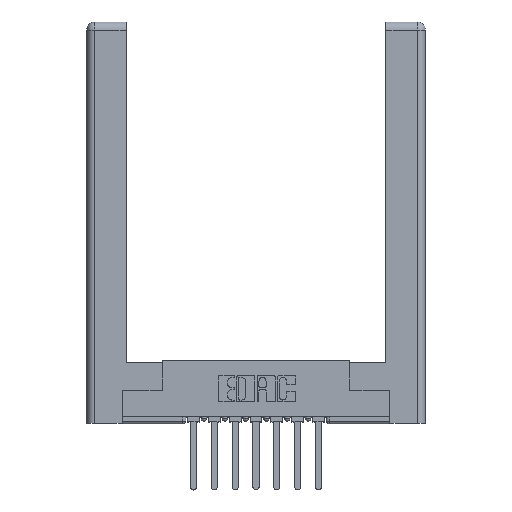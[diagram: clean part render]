
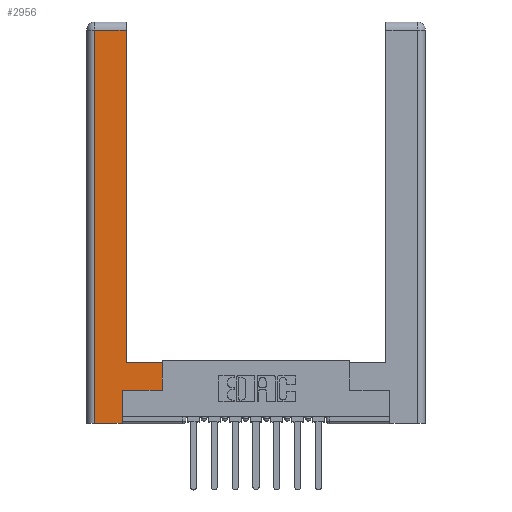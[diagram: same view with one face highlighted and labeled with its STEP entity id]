
A CAD part, top view. The second image highlights one B-rep face of the part: STEP entity #2956.
In plain terms, the highlighted planar face has unit normal (0, 0, 1).
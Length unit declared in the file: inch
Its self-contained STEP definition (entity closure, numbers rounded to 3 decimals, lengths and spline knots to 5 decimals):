
#50 = DIRECTION ( 'NONE',  ( -1., 0., 0. ) ) ;
#137 = DIRECTION ( 'NONE',  ( 0., 1., 0. ) ) ;
#250 = CARTESIAN_POINT ( 'NONE',  ( 0.265, 0.245, 0. ) ) ;
#469 = CARTESIAN_POINT ( 'NONE',  ( 0.295, 2.94, 0. ) ) ;
#1010 = VERTEX_POINT ( 'NONE', #1948 ) ;
#1033 = ORIENTED_EDGE ( 'NONE', *, *, #1061, .T. ) ;
#1061 = EDGE_CURVE ( 'NONE', #2699, #8455, #7199, .T. ) ;
#1087 = VERTEX_POINT ( 'NONE', #6345 ) ;
#1153 = CARTESIAN_POINT ( 'NONE',  ( 0.0615, 0., 0. ) ) ;
#1284 = CARTESIAN_POINT ( 'NONE',  ( 0.265, 0., 0. ) ) ;
#1726 = DIRECTION ( 'NONE',  ( 1., 0., 0. ) ) ;
#1829 = ORIENTED_EDGE ( 'NONE', *, *, #2673, .T. ) ;
#1948 = CARTESIAN_POINT ( 'NONE',  ( 0.295, 0.45, 0. ) ) ;
#2093 = VECTOR ( 'NONE', #1726, 39.37008 ) ;
#2288 = DIRECTION ( 'NONE',  ( -1., 0., 0. ) ) ;
#2411 = LINE ( 'NONE', #10979, #10341 ) ;
#2460 = VECTOR ( 'NONE', #11695, 39.37008 ) ;
#2673 = EDGE_CURVE ( 'NONE', #10472, #10853, #9185, .T. ) ;
#2699 = VERTEX_POINT ( 'NONE', #469 ) ;
#2748 = CARTESIAN_POINT ( 'NONE',  ( 0.265, 0.245, 0. ) ) ;
#2874 = VECTOR ( 'NONE', #50, 39.37008 ) ;
#2956 = ADVANCED_FACE ( 'NONE', ( #8522 ), #5592, .F. ) ;
#3079 = CARTESIAN_POINT ( 'NONE',  ( 0.295, 0.45, 0. ) ) ;
#3180 = EDGE_CURVE ( 'NONE', #10853, #1087, #10027, .T. ) ;
#3404 = DIRECTION ( 'NONE',  ( 0., 1., 0. ) ) ;
#3764 = ORIENTED_EDGE ( 'NONE', *, *, #3180, .T. ) ;
#3773 = CARTESIAN_POINT ( 'NONE',  ( 0.565, 0.245, 0. ) ) ;
#4238 = VECTOR ( 'NONE', #2288, 39.37008 ) ;
#4495 = DIRECTION ( 'NONE',  ( 0., 1., 0. ) ) ;
#4702 = AXIS2_PLACEMENT_3D ( 'NONE', #13193, #13067, #6669 ) ;
#4925 = LINE ( 'NONE', #6634, #10944 ) ;
#5345 = ORIENTED_EDGE ( 'NONE', *, *, #11799, .T. ) ;
#5592 = PLANE ( 'NONE',  #4702 ) ;
#5763 = ORIENTED_EDGE ( 'NONE', *, *, #10010, .T. ) ;
#6034 = LINE ( 'NONE', #1153, #2460 ) ;
#6285 = DIRECTION ( 'NONE',  ( 1., 0., 0. ) ) ;
#6345 = CARTESIAN_POINT ( 'NONE',  ( 0.565, 0.245, 0. ) ) ;
#6634 = CARTESIAN_POINT ( 'NONE',  ( 0.565, 0.45, 0. ) ) ;
#6669 = DIRECTION ( 'NONE',  ( -1., 0., 0. ) ) ;
#7048 = ORIENTED_EDGE ( 'NONE', *, *, #7318, .T. ) ;
#7199 = LINE ( 'NONE', #11813, #4238 ) ;
#7318 = EDGE_CURVE ( 'NONE', #12815, #1010, #11314, .T. ) ;
#7414 = CARTESIAN_POINT ( 'NONE',  ( 0.295, 3., 0. ) ) ;
#7837 = ORIENTED_EDGE ( 'NONE', *, *, #11173, .T. ) ;
#8182 = VECTOR ( 'NONE', #4495, 39.37008 ) ;
#8455 = VERTEX_POINT ( 'NONE', #13399 ) ;
#8522 = FACE_OUTER_BOUND ( 'NONE', #13096, .T. ) ;
#8651 = VERTEX_POINT ( 'NONE', #12934 ) ;
#8789 = EDGE_CURVE ( 'NONE', #1087, #12815, #4925, .T. ) ;
#9185 = LINE ( 'NONE', #250, #8182 ) ;
#10010 = EDGE_CURVE ( 'NONE', #8455, #8651, #6034, .T. ) ;
#10027 = LINE ( 'NONE', #3773, #2093 ) ;
#10341 = VECTOR ( 'NONE', #6285, 39.37008 ) ;
#10355 = VECTOR ( 'NONE', #137, 39.37008 ) ;
#10472 = VERTEX_POINT ( 'NONE', #1284 ) ;
#10853 = VERTEX_POINT ( 'NONE', #2748 ) ;
#10944 = VECTOR ( 'NONE', #3404, 39.37008 ) ;
#10979 = CARTESIAN_POINT ( 'NONE',  ( 0.265, 0., 0. ) ) ;
#11042 = LINE ( 'NONE', #7414, #10355 ) ;
#11173 = EDGE_CURVE ( 'NONE', #1010, #2699, #11042, .T. ) ;
#11314 = LINE ( 'NONE', #3079, #2874 ) ;
#11541 = ORIENTED_EDGE ( 'NONE', *, *, #8789, .T. ) ;
#11695 = DIRECTION ( 'NONE',  ( 0., -1., 0. ) ) ;
#11799 = EDGE_CURVE ( 'NONE', #8651, #10472, #2411, .T. ) ;
#11813 = CARTESIAN_POINT ( 'NONE',  ( 0.0615, 2.94, 0. ) ) ;
#12571 = CARTESIAN_POINT ( 'NONE',  ( 0.565, 0.45, 0. ) ) ;
#12815 = VERTEX_POINT ( 'NONE', #12571 ) ;
#12934 = CARTESIAN_POINT ( 'NONE',  ( 0.0615, 0., 0. ) ) ;
#13067 = DIRECTION ( 'NONE',  ( 0., 0., -1. ) ) ;
#13096 = EDGE_LOOP ( 'NONE', ( #7837, #1033, #5763, #5345, #1829, #3764, #11541, #7048 ) ) ;
#13193 = CARTESIAN_POINT ( 'NONE',  ( 0., 0., 0. ) ) ;
#13399 = CARTESIAN_POINT ( 'NONE',  ( 0.0615, 2.94, 0. ) ) ;
